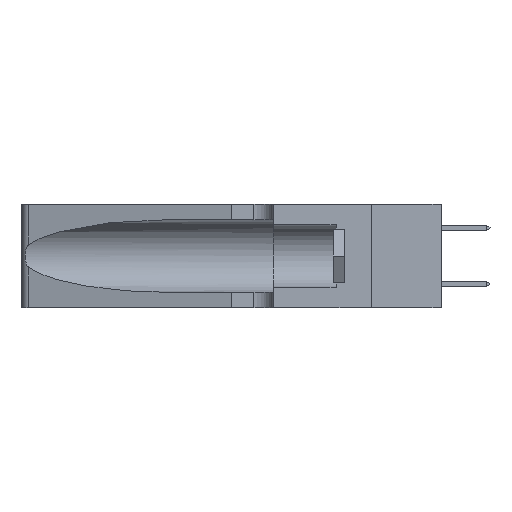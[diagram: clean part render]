
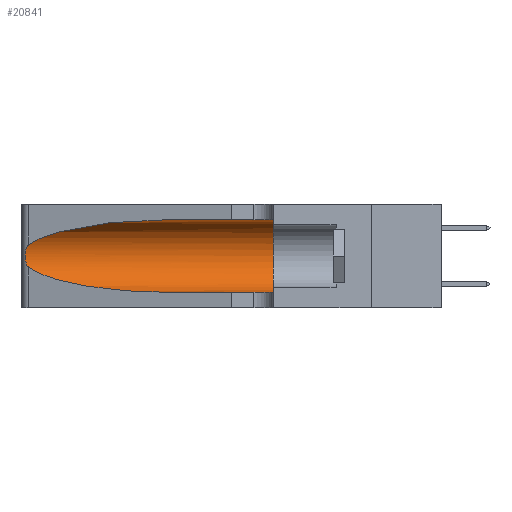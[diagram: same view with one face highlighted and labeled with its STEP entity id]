
A CAD part, left-side view. The second image highlights one B-rep face of the part: STEP entity #20841.
In plain terms, the highlighted cylindrical face has radius 3.308 mm (diameter 6.617 mm), a partial arc.
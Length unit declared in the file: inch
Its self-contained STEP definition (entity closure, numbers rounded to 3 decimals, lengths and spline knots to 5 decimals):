
#164 = VERTEX_POINT ( 'NONE', #25140 ) ;
#166 = FACE_OUTER_BOUND ( 'NONE', #27262, .T. ) ;
#660 = CARTESIAN_POINT ( 'NONE',  ( 0.1305, 0.35, 0.185 ) ) ;
#734 = CARTESIAN_POINT ( 'NONE',  ( 0.25487, 1.22718, 0.22369 ) ) ;
#747 = DIRECTION ( 'NONE',  ( 0., -1., 0. ) ) ;
#1036 = EDGE_CURVE ( 'NONE', #25415, #13251, #5195, .T. ) ;
#1213 = CARTESIAN_POINT ( 'NONE',  ( 0.25856, 1.23593, 0.16098 ) ) ;
#2920 = ORIENTED_EDGE ( 'NONE', *, *, #1036, .F. ) ;
#3339 = CARTESIAN_POINT ( 'NONE',  ( 0.26075, 1.23896, 0.178 ) ) ;
#3525 = CARTESIAN_POINT ( 'NONE',  ( 0.25639, 1.23184, 0.21858 ) ) ;
#3610 = CARTESIAN_POINT ( 'NONE',  ( 0.25555, 1.22993, 0.14849 ) ) ;
#3940 = DIRECTION ( 'NONE',  ( 0., -1., 0. ) ) ;
#4389 = CARTESIAN_POINT ( 'NONE',  ( 0.1305, 0.35, 0.05475 ) ) ;
#4407 = ORIENTED_EDGE ( 'NONE', *, *, #19972, .T. ) ;
#4523 = CARTESIAN_POINT ( 'NONE',  ( 0.1305, 1.61858, 0.185 ) ) ;
#4892 = DIRECTION ( 'NONE',  ( 0., 0., 1. ) ) ;
#5195 = LINE ( 'NONE', #25293, #19447 ) ;
#6150 = CARTESIAN_POINT ( 'NONE',  ( 0.25487, 1.22718, 0.22369 ) ) ;
#6860 = LINE ( 'NONE', #10584, #17150 ) ;
#6864 = DIRECTION ( 'NONE',  ( 0., 1., 0. ) ) ;
#7495 = CARTESIAN_POINT ( 'NONE',  ( 0.26017, 1.23833, 0.17102 ) ) ;
#9572 = ORIENTED_EDGE ( 'NONE', *, *, #13753, .T. ) ;
#10087 =( BOUNDED_CURVE ( )  B_SPLINE_CURVE ( 3, ( #16888, #19105, #23347, #6150 ),
 .UNSPECIFIED., .F., .T. ) 
 B_SPLINE_CURVE_WITH_KNOTS ( ( 4, 4 ),
 ( 1.5708, 2.84003 ),
 .UNSPECIFIED. ) 
 CURVE ( )  GEOMETRIC_REPRESENTATION_ITEM ( )  RATIONAL_B_SPLINE_CURVE ( ( 1., 0.87, 0.87, 1. ) ) 
 REPRESENTATION_ITEM ( '' )  );
#10584 = CARTESIAN_POINT ( 'NONE',  ( 0.1305, 1.61858, 0.05475 ) ) ;
#10698 = CARTESIAN_POINT ( 'NONE',  ( 0.25487, 1.22718, 0.14631 ) ) ;
#10791 = CARTESIAN_POINT ( 'NONE',  ( 0.18966, 0.96281, 0.05475 ) ) ;
#10883 = CARTESIAN_POINT ( 'NONE',  ( 0.2373, 1.15595, 0.08982 ) ) ;
#11819 = CARTESIAN_POINT ( 'NONE',  ( 0.25487, 1.22718, 0.14631 ) ) ;
#11912 = CARTESIAN_POINT ( 'NONE',  ( 0.25789, 1.23486, 0.15765 ) ) ;
#12105 = CARTESIAN_POINT ( 'NONE',  ( 0.25555, 1.22994, 0.2215 ) ) ;
#12122 =( BOUNDED_CURVE ( )  B_SPLINE_CURVE ( 3, ( #10698, #10883, #10791, #25364 ),
 .UNSPECIFIED., .F., .T. ) 
 B_SPLINE_CURVE_WITH_KNOTS ( ( 4, 4 ),
 ( 3.44316, 4.71239 ),
 .UNSPECIFIED. ) 
 CURVE ( )  GEOMETRIC_REPRESENTATION_ITEM ( )  RATIONAL_B_SPLINE_CURVE ( ( 1., 0.87, 0.87, 1. ) ) 
 REPRESENTATION_ITEM ( '' )  );
#12727 = CARTESIAN_POINT ( 'NONE',  ( 0.25487, 1.22718, 0.14631 ) ) ;
#12843 = CARTESIAN_POINT ( 'NONE',  ( 0.1305, 0.72297, 0.31525 ) ) ;
#13246 = EDGE_CURVE ( 'NONE', #13251, #18729, #20406, .T. ) ;
#13251 = VERTEX_POINT ( 'NONE', #13318 ) ;
#13318 = CARTESIAN_POINT ( 'NONE',  ( 0.1305, 0.35, 0.31525 ) ) ;
#13753 = EDGE_CURVE ( 'NONE', #16290, #164, #12122, .T. ) ;
#15340 = ORIENTED_EDGE ( 'NONE', *, *, #21139, .T. ) ;
#15361 = ORIENTED_EDGE ( 'NONE', *, *, #22491, .T. ) ;
#16147 = AXIS2_PLACEMENT_3D ( 'NONE', #660, #6864, #4892 ) ;
#16290 = VERTEX_POINT ( 'NONE', #12727 ) ;
#16888 = CARTESIAN_POINT ( 'NONE',  ( 0.1305, 0.72297, 0.31525 ) ) ;
#17150 = VECTOR ( 'NONE', #3940, 39.37008 ) ;
#17498 = DIRECTION ( 'NONE',  ( 0., 0., -1. ) ) ;
#18430 = CARTESIAN_POINT ( 'NONE',  ( 0.25854, 1.2359, 0.20912 ) ) ;
#18729 = VERTEX_POINT ( 'NONE', #4389 ) ;
#19105 = CARTESIAN_POINT ( 'NONE',  ( 0.18966, 0.96281, 0.31525 ) ) ;
#19447 = VECTOR ( 'NONE', #747, 39.37008 ) ;
#19945 = B_SPLINE_CURVE_WITH_KNOTS ( 'NONE', 3,
 ( #20188, #12105, #3525, #22422, #18430, #26697, #20486, #3339, #7495, #1213, #11912, #20289, #3610, #11819 ),
 .UNSPECIFIED., .F., .F.,
 ( 4, 2, 2, 2, 2, 2, 4 ),
 ( 0., 0.00027, 0.00053, 0.00107, 0.0016, 0.00187, 0.00214 ),
 .UNSPECIFIED. ) ;
#19972 = EDGE_CURVE ( 'NONE', #164, #18729, #6860, .T. ) ;
#20188 = CARTESIAN_POINT ( 'NONE',  ( 0.25487, 1.22718, 0.22369 ) ) ;
#20289 = CARTESIAN_POINT ( 'NONE',  ( 0.25639, 1.23186, 0.15144 ) ) ;
#20406 = CIRCLE ( 'NONE', #16147, 0.13025 ) ;
#20480 = ORIENTED_EDGE ( 'NONE', *, *, #13246, .F. ) ;
#20486 = CARTESIAN_POINT ( 'NONE',  ( 0.26075, 1.23896, 0.19203 ) ) ;
#20841 = ADVANCED_FACE ( 'NONE', ( #166 ), #22398, .F. ) ;
#21139 = EDGE_CURVE ( 'NONE', #23243, #16290, #19945, .T. ) ;
#22236 = AXIS2_PLACEMENT_3D ( 'NONE', #4523, #23606, #17498 ) ;
#22398 = CYLINDRICAL_SURFACE ( 'NONE', #22236, 0.13025 ) ;
#22422 = CARTESIAN_POINT ( 'NONE',  ( 0.25787, 1.23484, 0.2124 ) ) ;
#22491 = EDGE_CURVE ( 'NONE', #25415, #23243, #10087, .T. ) ;
#23243 = VERTEX_POINT ( 'NONE', #734 ) ;
#23347 = CARTESIAN_POINT ( 'NONE',  ( 0.2373, 1.15595, 0.28018 ) ) ;
#23606 = DIRECTION ( 'NONE',  ( 0., -1., 0. ) ) ;
#25140 = CARTESIAN_POINT ( 'NONE',  ( 0.1305, 0.72297, 0.05475 ) ) ;
#25293 = CARTESIAN_POINT ( 'NONE',  ( 0.1305, 1.61858, 0.31525 ) ) ;
#25364 = CARTESIAN_POINT ( 'NONE',  ( 0.1305, 0.72297, 0.05475 ) ) ;
#25415 = VERTEX_POINT ( 'NONE', #12843 ) ;
#26697 = CARTESIAN_POINT ( 'NONE',  ( 0.26018, 1.23835, 0.19895 ) ) ;
#27262 = EDGE_LOOP ( 'NONE', ( #15361, #15340, #9572, #4407, #20480, #2920 ) ) ;
